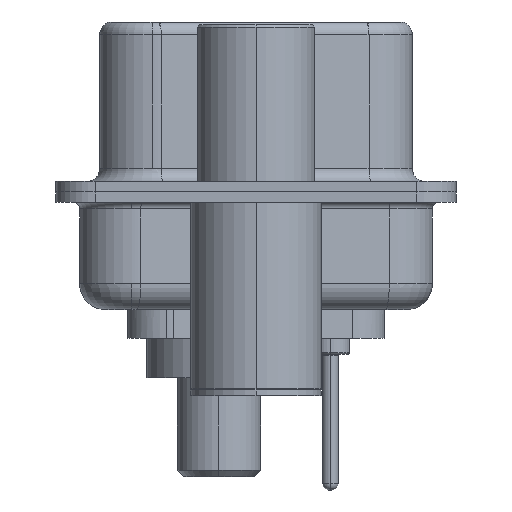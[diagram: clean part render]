
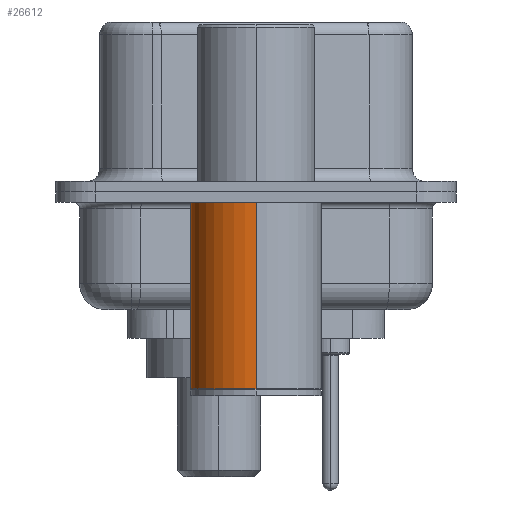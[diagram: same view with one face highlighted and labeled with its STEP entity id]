
A CAD part, left-side view. The second image highlights one B-rep face of the part: STEP entity #26612.
In plain terms, the highlighted cylindrical face has radius 2.5 mm (diameter 5 mm), a partial arc.
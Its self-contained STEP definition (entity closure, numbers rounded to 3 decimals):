
#103 = LINE ( 'NONE', #21425, #5235 ) ;
#1145 = EDGE_CURVE ( 'NONE', #6982, #15290, #27184, .T. ) ;
#3259 = DIRECTION ( 'NONE',  ( 0., 0., 1. ) ) ;
#3694 = EDGE_CURVE ( 'NONE', #9932, #27041, #24040, .T. ) ;
#3876 = AXIS2_PLACEMENT_3D ( 'NONE', #20622, #3259, #16347 ) ;
#4229 = AXIS2_PLACEMENT_3D ( 'NONE', #8774, #7297, #21271 ) ;
#5148 = ORIENTED_EDGE ( 'NONE', *, *, #16696, .F. ) ;
#5235 = VECTOR ( 'NONE', #10475, 1000. ) ;
#5883 = CYLINDRICAL_SURFACE ( 'NONE', #3876, 2.5 ) ;
#6982 = VERTEX_POINT ( 'NONE', #27098 ) ;
#7297 = DIRECTION ( 'NONE',  ( 0., 0., 1. ) ) ;
#7902 = CARTESIAN_POINT ( 'NONE',  ( -2.5, 0., 0.581 ) ) ;
#8774 = CARTESIAN_POINT ( 'NONE',  ( 0., 0., -7.525 ) ) ;
#9571 = CARTESIAN_POINT ( 'NONE',  ( 0., 0., -0.4 ) ) ;
#9932 = VERTEX_POINT ( 'NONE', #19638 ) ;
#10064 = DIRECTION ( 'NONE',  ( 0., 0., 1. ) ) ;
#10397 = DIRECTION ( 'NONE',  ( 0., 0., 1. ) ) ;
#10475 = DIRECTION ( 'NONE',  ( 0., 0., 1. ) ) ;
#11177 = ORIENTED_EDGE ( 'NONE', *, *, #1145, .F. ) ;
#11942 = EDGE_CURVE ( 'NONE', #27041, #15290, #23754, .T. ) ;
#15290 = VERTEX_POINT ( 'NONE', #27619 ) ;
#16347 = DIRECTION ( 'NONE',  ( 1., 0., 0. ) ) ;
#16696 = EDGE_CURVE ( 'NONE', #9932, #6982, #103, .T. ) ;
#17461 = FACE_OUTER_BOUND ( 'NONE', #24696, .T. ) ;
#17798 = DIRECTION ( 'NONE',  ( 1., 0., 0. ) ) ;
#17920 = VECTOR ( 'NONE', #10064, 1000. ) ;
#19638 = CARTESIAN_POINT ( 'NONE',  ( 2.5, 0., -7.525 ) ) ;
#20622 = CARTESIAN_POINT ( 'NONE',  ( 0., 0., 0.581 ) ) ;
#21271 = DIRECTION ( 'NONE',  ( 1., 0., 0. ) ) ;
#21425 = CARTESIAN_POINT ( 'NONE',  ( 2.5, 0., 0.581 ) ) ;
#23566 = ORIENTED_EDGE ( 'NONE', *, *, #11942, .T. ) ;
#23754 = LINE ( 'NONE', #7902, #17920 ) ;
#24040 = CIRCLE ( 'NONE', #4229, 2.5 ) ;
#24696 = EDGE_LOOP ( 'NONE', ( #25799, #23566, #11177, #5148 ) ) ;
#25799 = ORIENTED_EDGE ( 'NONE', *, *, #3694, .T. ) ;
#26612 = ADVANCED_FACE ( 'NONE', ( #17461 ), #5883, .T. ) ;
#26766 = CARTESIAN_POINT ( 'NONE',  ( -2.5, 0., -7.525 ) ) ;
#27041 = VERTEX_POINT ( 'NONE', #26766 ) ;
#27098 = CARTESIAN_POINT ( 'NONE',  ( 2.5, 0., -0.4 ) ) ;
#27184 = CIRCLE ( 'NONE', #28134, 2.5 ) ;
#27619 = CARTESIAN_POINT ( 'NONE',  ( -2.5, 0., -0.4 ) ) ;
#28134 = AXIS2_PLACEMENT_3D ( 'NONE', #9571, #10397, #17798 ) ;
